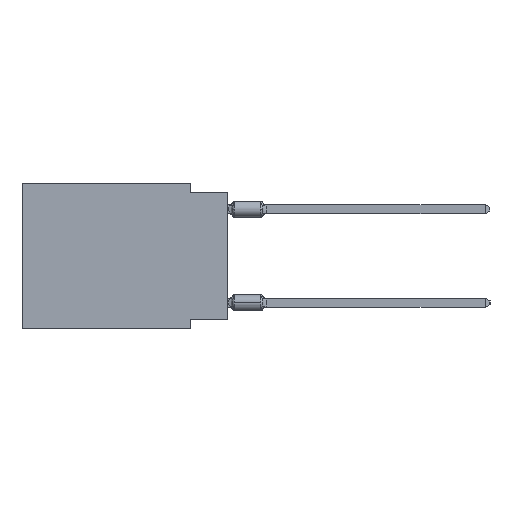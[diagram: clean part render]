
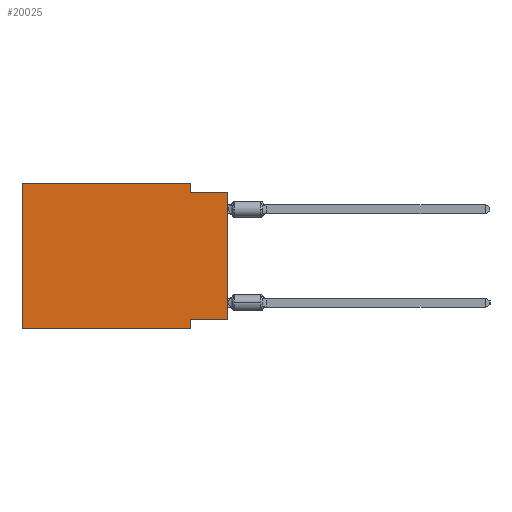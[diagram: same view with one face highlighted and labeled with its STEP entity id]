
A CAD part, left-side view. The second image highlights one B-rep face of the part: STEP entity #20025.
In plain terms, the highlighted planar face has unit normal (-1, 0, 0).
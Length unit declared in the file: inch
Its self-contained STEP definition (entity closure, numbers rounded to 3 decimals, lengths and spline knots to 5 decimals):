
#245 = LINE ( 'NONE', #35652, #6312 ) ;
#259 = LINE ( 'NONE', #13356, #18417 ) ;
#472 = ORIENTED_EDGE ( 'NONE', *, *, #36159, .T. ) ;
#1362 = CARTESIAN_POINT ( 'NONE',  ( 0., 0.1, -0.39 ) ) ;
#2295 = CARTESIAN_POINT ( 'NONE',  ( 0., 0.1, -0.365 ) ) ;
#2560 = DIRECTION ( 'NONE',  ( 0., 1., 0. ) ) ;
#2731 = EDGE_CURVE ( 'NONE', #36014, #19260, #7544, .T. ) ;
#4181 = VECTOR ( 'NONE', #29844, 39.37008 ) ;
#4244 = LINE ( 'NONE', #17539, #24124 ) ;
#4350 = EDGE_LOOP ( 'NONE', ( #472, #25615, #11089, #37384, #26901, #26764, #38403, #4793 ) ) ;
#4793 = ORIENTED_EDGE ( 'NONE', *, *, #2731, .F. ) ;
#6154 = VECTOR ( 'NONE', #2560, 39.37008 ) ;
#6298 = EDGE_CURVE ( 'NONE', #32629, #35161, #259, .T. ) ;
#6312 = VECTOR ( 'NONE', #13118, 39.37008 ) ;
#6580 = LINE ( 'NONE', #22693, #32930 ) ;
#7141 = EDGE_CURVE ( 'NONE', #23915, #24686, #4244, .T. ) ;
#7544 = LINE ( 'NONE', #11593, #6154 ) ;
#9251 = CARTESIAN_POINT ( 'NONE',  ( 0., 0.1, -0.39 ) ) ;
#10112 = VECTOR ( 'NONE', #14444, 39.37008 ) ;
#10117 = DIRECTION ( 'NONE',  ( 0., -1., 0. ) ) ;
#10136 = CARTESIAN_POINT ( 'NONE',  ( 0., 0.55, -0.39 ) ) ;
#11089 = ORIENTED_EDGE ( 'NONE', *, *, #41562, .F. ) ;
#11334 = VERTEX_POINT ( 'NONE', #9251 ) ;
#11593 = CARTESIAN_POINT ( 'NONE',  ( 0., 0., -0.365 ) ) ;
#12308 = EDGE_CURVE ( 'NONE', #19260, #11334, #20912, .T. ) ;
#13118 = DIRECTION ( 'NONE',  ( 0., 0., -1. ) ) ;
#13356 = CARTESIAN_POINT ( 'NONE',  ( 0., 0.55, 0. ) ) ;
#13520 = PLANE ( 'NONE',  #13633 ) ;
#13633 = AXIS2_PLACEMENT_3D ( 'NONE', #33262, #26180, #36909 ) ;
#13751 = CARTESIAN_POINT ( 'NONE',  ( 0., 0.55, 0. ) ) ;
#14444 = DIRECTION ( 'NONE',  ( 0., 0., -1. ) ) ;
#14648 = FACE_OUTER_BOUND ( 'NONE', #4350, .T. ) ;
#15200 = CARTESIAN_POINT ( 'NONE',  ( 0., 0.1, 0. ) ) ;
#17128 = CARTESIAN_POINT ( 'NONE',  ( 0., 0., -0.025 ) ) ;
#17539 = CARTESIAN_POINT ( 'NONE',  ( 0., 0., -0.025 ) ) ;
#18417 = VECTOR ( 'NONE', #10117, 39.37008 ) ;
#18495 = CARTESIAN_POINT ( 'NONE',  ( 0., 0., -0.365 ) ) ;
#19260 = VERTEX_POINT ( 'NONE', #2295 ) ;
#20025 = ADVANCED_FACE ( 'NONE', ( #14648 ), #13520, .F. ) ;
#20912 = LINE ( 'NONE', #1362, #10112 ) ;
#21763 = EDGE_CURVE ( 'NONE', #35666, #11334, #6580, .T. ) ;
#21802 = CARTESIAN_POINT ( 'NONE',  ( 0., 0.55, 0. ) ) ;
#22361 = DIRECTION ( 'NONE',  ( 0., 0., 1. ) ) ;
#22693 = CARTESIAN_POINT ( 'NONE',  ( 0., 0.55, -0.39 ) ) ;
#23915 = VERTEX_POINT ( 'NONE', #30086 ) ;
#24124 = VECTOR ( 'NONE', #40698, 39.37008 ) ;
#24686 = VERTEX_POINT ( 'NONE', #17128 ) ;
#24815 = VECTOR ( 'NONE', #22361, 39.37008 ) ;
#25148 = CARTESIAN_POINT ( 'NONE',  ( 0., 0., 0. ) ) ;
#25615 = ORIENTED_EDGE ( 'NONE', *, *, #7141, .F. ) ;
#25897 = DIRECTION ( 'NONE',  ( 0., -1., 0. ) ) ;
#26180 = DIRECTION ( 'NONE',  ( 1., 0., 0. ) ) ;
#26764 = ORIENTED_EDGE ( 'NONE', *, *, #21763, .T. ) ;
#26901 = ORIENTED_EDGE ( 'NONE', *, *, #34963, .F. ) ;
#29844 = DIRECTION ( 'NONE',  ( 0., 0., 1. ) ) ;
#30086 = CARTESIAN_POINT ( 'NONE',  ( 0., 0.1, -0.025 ) ) ;
#30488 = LINE ( 'NONE', #13751, #4181 ) ;
#32629 = VERTEX_POINT ( 'NONE', #21802 ) ;
#32930 = VECTOR ( 'NONE', #25897, 39.37008 ) ;
#33262 = CARTESIAN_POINT ( 'NONE',  ( 0., 0.55, 0. ) ) ;
#34963 = EDGE_CURVE ( 'NONE', #35666, #32629, #30488, .T. ) ;
#35161 = VERTEX_POINT ( 'NONE', #15200 ) ;
#35652 = CARTESIAN_POINT ( 'NONE',  ( 0., 0.1, 0. ) ) ;
#35666 = VERTEX_POINT ( 'NONE', #10136 ) ;
#36014 = VERTEX_POINT ( 'NONE', #18495 ) ;
#36159 = EDGE_CURVE ( 'NONE', #36014, #24686, #40675, .T. ) ;
#36909 = DIRECTION ( 'NONE',  ( 0., 0., -1. ) ) ;
#37384 = ORIENTED_EDGE ( 'NONE', *, *, #6298, .F. ) ;
#38403 = ORIENTED_EDGE ( 'NONE', *, *, #12308, .F. ) ;
#40675 = LINE ( 'NONE', #25148, #24815 ) ;
#40698 = DIRECTION ( 'NONE',  ( 0., -1., 0. ) ) ;
#41562 = EDGE_CURVE ( 'NONE', #35161, #23915, #245, .T. ) ;
